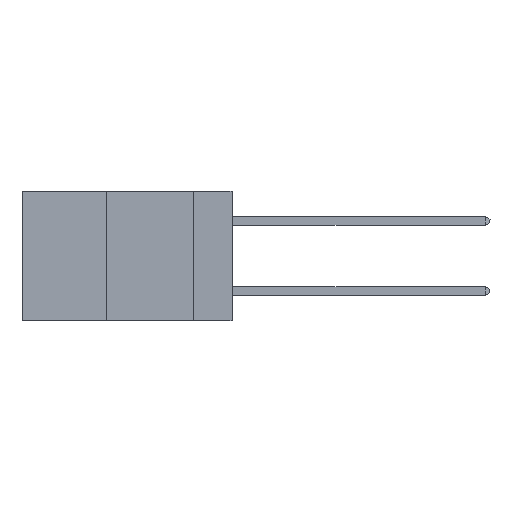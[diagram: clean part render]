
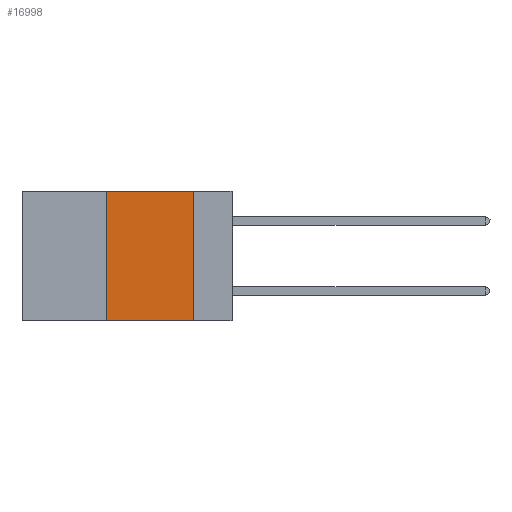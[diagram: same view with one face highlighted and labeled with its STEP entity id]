
A CAD part, left-side view. The second image highlights one B-rep face of the part: STEP entity #16998.
In plain terms, the highlighted planar face has unit normal (-1, 0, 0).
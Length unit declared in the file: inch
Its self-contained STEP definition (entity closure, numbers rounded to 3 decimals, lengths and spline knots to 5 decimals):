
#583 = CARTESIAN_POINT ( 'NONE',  ( 0., 0.6, 0. ) ) ;
#2192 = CARTESIAN_POINT ( 'NONE',  ( 0., 0.36, -0.37 ) ) ;
#2330 = EDGE_LOOP ( 'NONE', ( #17647, #19496, #7955, #3487 ) ) ;
#3371 = VERTEX_POINT ( 'NONE', #2192 ) ;
#3487 = ORIENTED_EDGE ( 'NONE', *, *, #18978, .T. ) ;
#3613 = FACE_OUTER_BOUND ( 'NONE', #2330, .T. ) ;
#4345 = CARTESIAN_POINT ( 'NONE',  ( 0., 0.6, -0.37 ) ) ;
#4677 = EDGE_CURVE ( 'NONE', #3371, #8905, #17806, .T. ) ;
#4959 = CARTESIAN_POINT ( 'NONE',  ( 0., 0.36, 0. ) ) ;
#5912 = EDGE_CURVE ( 'NONE', #15640, #18459, #11301, .T. ) ;
#6755 = CARTESIAN_POINT ( 'NONE',  ( 0., 0.11, 0. ) ) ;
#7955 = ORIENTED_EDGE ( 'NONE', *, *, #4677, .F. ) ;
#8905 = VERTEX_POINT ( 'NONE', #4959 ) ;
#9321 = CARTESIAN_POINT ( 'NONE',  ( 0., 0.36, 0. ) ) ;
#9758 = VECTOR ( 'NONE', #19388, 39.37008 ) ;
#9868 = CARTESIAN_POINT ( 'NONE',  ( 0., 0.6, 0. ) ) ;
#11190 = LINE ( 'NONE', #9868, #16870 ) ;
#11245 = EDGE_CURVE ( 'NONE', #8905, #15640, #11190, .T. ) ;
#11301 = LINE ( 'NONE', #16627, #9758 ) ;
#11523 = DIRECTION ( 'NONE',  ( 0., -1., 0. ) ) ;
#12114 = DIRECTION ( 'NONE',  ( 0., 0., -1. ) ) ;
#12139 = AXIS2_PLACEMENT_3D ( 'NONE', #583, #18524, #12114 ) ;
#12596 = CARTESIAN_POINT ( 'NONE',  ( 0., 0.11, -0.37 ) ) ;
#13957 = VECTOR ( 'NONE', #20803, 39.37008 ) ;
#15640 = VERTEX_POINT ( 'NONE', #6755 ) ;
#15801 = DIRECTION ( 'NONE',  ( 0., -1., 0. ) ) ;
#16627 = CARTESIAN_POINT ( 'NONE',  ( 0., 0.11, 0. ) ) ;
#16870 = VECTOR ( 'NONE', #11523, 39.37008 ) ;
#16894 = LINE ( 'NONE', #4345, #17424 ) ;
#16998 = ADVANCED_FACE ( 'NONE', ( #3613 ), #18661, .F. ) ;
#17424 = VECTOR ( 'NONE', #15801, 39.37008 ) ;
#17647 = ORIENTED_EDGE ( 'NONE', *, *, #5912, .F. ) ;
#17806 = LINE ( 'NONE', #9321, #13957 ) ;
#18459 = VERTEX_POINT ( 'NONE', #12596 ) ;
#18524 = DIRECTION ( 'NONE',  ( 1., 0., 0. ) ) ;
#18661 = PLANE ( 'NONE',  #12139 ) ;
#18978 = EDGE_CURVE ( 'NONE', #3371, #18459, #16894, .T. ) ;
#19388 = DIRECTION ( 'NONE',  ( 0., 0., -1. ) ) ;
#19496 = ORIENTED_EDGE ( 'NONE', *, *, #11245, .F. ) ;
#20803 = DIRECTION ( 'NONE',  ( 0., 0., 1. ) ) ;
